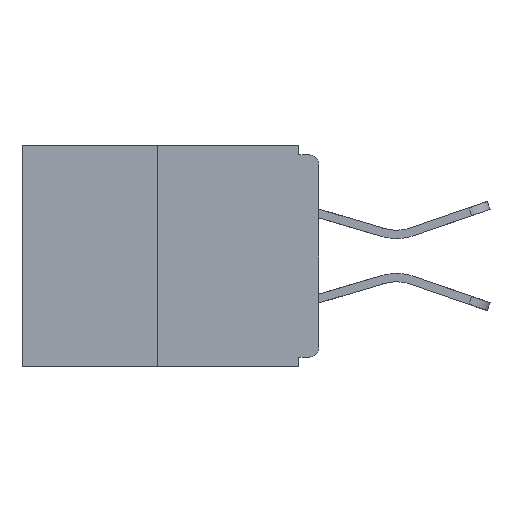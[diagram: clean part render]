
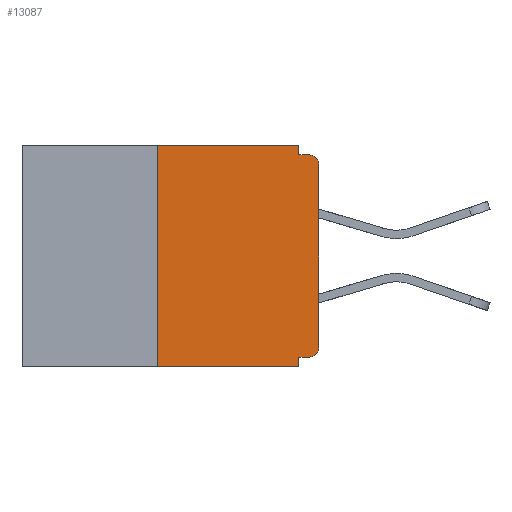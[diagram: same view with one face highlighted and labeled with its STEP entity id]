
A CAD part, left-side view. The second image highlights one B-rep face of the part: STEP entity #13087.
In plain terms, the highlighted planar face has unit normal (-1, 0, 0).
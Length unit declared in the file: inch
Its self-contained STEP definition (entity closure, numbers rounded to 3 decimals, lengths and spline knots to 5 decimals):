
#93 = EDGE_CURVE ( 'NONE', #383, #15744, #5281, .T. ) ;
#195 = CARTESIAN_POINT ( 'NONE',  ( 0., 0., -0.328 ) ) ;
#215 = CARTESIAN_POINT ( 'NONE',  ( 0., 0.015, -0.328 ) ) ;
#262 = LINE ( 'NONE', #5574, #11350 ) ;
#383 = VERTEX_POINT ( 'NONE', #4326 ) ;
#585 = VECTOR ( 'NONE', #1546, 39.37008 ) ;
#1167 = LINE ( 'NONE', #195, #7037 ) ;
#1168 = CARTESIAN_POINT ( 'NONE',  ( 0., 0.031, -0.328 ) ) ;
#1230 = CARTESIAN_POINT ( 'NONE',  ( 0., 0., -0.313 ) ) ;
#1294 = CARTESIAN_POINT ( 'NONE',  ( 0., 0.031, 0. ) ) ;
#1546 = DIRECTION ( 'NONE',  ( 0., -1., 0. ) ) ;
#1553 = EDGE_LOOP ( 'NONE', ( #6167, #8425, #10948, #13098, #13551, #13699, #13831, #5990, #15533, #6110 ) ) ;
#1830 = LINE ( 'NONE', #11847, #9882 ) ;
#1978 = VECTOR ( 'NONE', #5149, 39.37008 ) ;
#2127 = EDGE_CURVE ( 'NONE', #13832, #12869, #1167, .T. ) ;
#2393 = CIRCLE ( 'NONE', #8154, 0.015 ) ;
#2473 = CARTESIAN_POINT ( 'NONE',  ( 0., 0.46, 0. ) ) ;
#2504 = EDGE_CURVE ( 'NONE', #4189, #10663, #12452, .T. ) ;
#2698 = VECTOR ( 'NONE', #14151, 39.37008 ) ;
#2752 = CARTESIAN_POINT ( 'NONE',  ( 0., 0., -0.03 ) ) ;
#3052 = FACE_OUTER_BOUND ( 'NONE', #1553, .T. ) ;
#3365 = AXIS2_PLACEMENT_3D ( 'NONE', #4341, #13392, #9566 ) ;
#3608 = VERTEX_POINT ( 'NONE', #4834 ) ;
#3695 = CARTESIAN_POINT ( 'NONE',  ( 0., 0.015, -0.03 ) ) ;
#3986 = DIRECTION ( 'NONE',  ( 0., 0., -1. ) ) ;
#3998 = CARTESIAN_POINT ( 'NONE',  ( 0., 0.46, -0.343 ) ) ;
#4189 = VERTEX_POINT ( 'NONE', #1230 ) ;
#4326 = CARTESIAN_POINT ( 'NONE',  ( 0., 0.25, -0.343 ) ) ;
#4341 = CARTESIAN_POINT ( 'NONE',  ( 0., 0.46, 0. ) ) ;
#4516 = EDGE_CURVE ( 'NONE', #13832, #4189, #13817, .T. ) ;
#4834 = CARTESIAN_POINT ( 'NONE',  ( 0., 0.031, -0.015 ) ) ;
#5149 = DIRECTION ( 'NONE',  ( 0., 0., 1. ) ) ;
#5281 = LINE ( 'NONE', #3998, #7721 ) ;
#5574 = CARTESIAN_POINT ( 'NONE',  ( 0., 0.031, 0. ) ) ;
#5889 = VERTEX_POINT ( 'NONE', #15450 ) ;
#5931 = EDGE_CURVE ( 'NONE', #11402, #8004, #10548, .T. ) ;
#5990 = ORIENTED_EDGE ( 'NONE', *, *, #14294, .T. ) ;
#6110 = ORIENTED_EDGE ( 'NONE', *, *, #12224, .F. ) ;
#6167 = ORIENTED_EDGE ( 'NONE', *, *, #5931, .F. ) ;
#6885 = DIRECTION ( 'NONE',  ( 0., 0., 1. ) ) ;
#7037 = VECTOR ( 'NONE', #10446, 39.37008 ) ;
#7721 = VECTOR ( 'NONE', #14127, 39.37008 ) ;
#7871 = CARTESIAN_POINT ( 'NONE',  ( 0., 0., 0. ) ) ;
#8004 = VERTEX_POINT ( 'NONE', #1294 ) ;
#8154 = AXIS2_PLACEMENT_3D ( 'NONE', #3695, #12645, #15296 ) ;
#8425 = ORIENTED_EDGE ( 'NONE', *, *, #9587, .F. ) ;
#9284 = CARTESIAN_POINT ( 'NONE',  ( 0., 0., -0.015 ) ) ;
#9434 = VECTOR ( 'NONE', #6885, 39.37008 ) ;
#9539 = AXIS2_PLACEMENT_3D ( 'NONE', #11726, #12857, #15624 ) ;
#9566 = DIRECTION ( 'NONE',  ( 0., 0., -1. ) ) ;
#9587 = EDGE_CURVE ( 'NONE', #383, #11402, #16298, .T. ) ;
#9882 = VECTOR ( 'NONE', #3986, 39.37008 ) ;
#10223 = EDGE_CURVE ( 'NONE', #12869, #15744, #1830, .T. ) ;
#10382 = CARTESIAN_POINT ( 'NONE',  ( 0., 0.031, -0.343 ) ) ;
#10446 = DIRECTION ( 'NONE',  ( 0., 1., 0. ) ) ;
#10548 = LINE ( 'NONE', #2473, #2698 ) ;
#10663 = VERTEX_POINT ( 'NONE', #2752 ) ;
#10948 = ORIENTED_EDGE ( 'NONE', *, *, #93, .T. ) ;
#11350 = VECTOR ( 'NONE', #14373, 39.37008 ) ;
#11402 = VERTEX_POINT ( 'NONE', #16664 ) ;
#11726 = CARTESIAN_POINT ( 'NONE',  ( 0., 0.015, -0.313 ) ) ;
#11847 = CARTESIAN_POINT ( 'NONE',  ( 0., 0.031, -0.343 ) ) ;
#12224 = EDGE_CURVE ( 'NONE', #8004, #3608, #262, .T. ) ;
#12452 = LINE ( 'NONE', #7871, #1978 ) ;
#12645 = DIRECTION ( 'NONE',  ( -1., 0., 0. ) ) ;
#12857 = DIRECTION ( 'NONE',  ( -1., 0., 0. ) ) ;
#12869 = VERTEX_POINT ( 'NONE', #1168 ) ;
#13087 = ADVANCED_FACE ( 'NONE', ( #3052 ), #13448, .F. ) ;
#13098 = ORIENTED_EDGE ( 'NONE', *, *, #10223, .F. ) ;
#13392 = DIRECTION ( 'NONE',  ( 1., 0., 0. ) ) ;
#13448 = PLANE ( 'NONE',  #3365 ) ;
#13551 = ORIENTED_EDGE ( 'NONE', *, *, #2127, .F. ) ;
#13699 = ORIENTED_EDGE ( 'NONE', *, *, #4516, .T. ) ;
#13817 = CIRCLE ( 'NONE', #9539, 0.015 ) ;
#13831 = ORIENTED_EDGE ( 'NONE', *, *, #2504, .T. ) ;
#13832 = VERTEX_POINT ( 'NONE', #215 ) ;
#14127 = DIRECTION ( 'NONE',  ( 0., -1., 0. ) ) ;
#14151 = DIRECTION ( 'NONE',  ( 0., -1., 0. ) ) ;
#14294 = EDGE_CURVE ( 'NONE', #10663, #5889, #2393, .T. ) ;
#14373 = DIRECTION ( 'NONE',  ( 0., 0., -1. ) ) ;
#14627 = EDGE_CURVE ( 'NONE', #3608, #5889, #15295, .T. ) ;
#15295 = LINE ( 'NONE', #9284, #585 ) ;
#15296 = DIRECTION ( 'NONE',  ( 0., 0., -1. ) ) ;
#15450 = CARTESIAN_POINT ( 'NONE',  ( 0., 0.015, -0.015 ) ) ;
#15533 = ORIENTED_EDGE ( 'NONE', *, *, #14627, .F. ) ;
#15624 = DIRECTION ( 'NONE',  ( 0., 0., -1. ) ) ;
#15744 = VERTEX_POINT ( 'NONE', #10382 ) ;
#15975 = CARTESIAN_POINT ( 'NONE',  ( 0., 0.25, 0. ) ) ;
#16298 = LINE ( 'NONE', #15975, #9434 ) ;
#16664 = CARTESIAN_POINT ( 'NONE',  ( 0., 0.25, 0. ) ) ;
